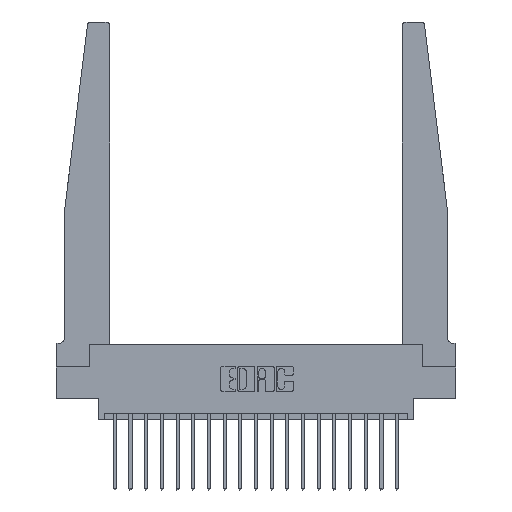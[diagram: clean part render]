
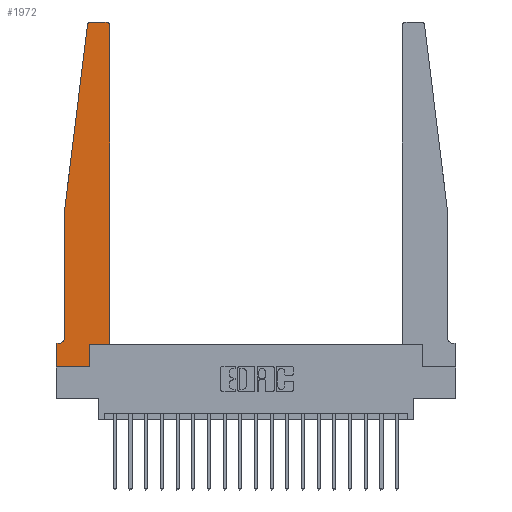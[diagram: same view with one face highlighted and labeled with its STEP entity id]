
A CAD part, top view. The second image highlights one B-rep face of the part: STEP entity #1972.
In plain terms, the highlighted planar face has unit normal (0, 0, 1).
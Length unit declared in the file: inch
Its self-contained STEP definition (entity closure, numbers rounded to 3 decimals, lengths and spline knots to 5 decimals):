
#54 = DIRECTION ( 'NONE',  ( 0., 0., -1. ) ) ;
#365 = VECTOR ( 'NONE', #19002, 39.37008 ) ;
#489 = EDGE_CURVE ( 'NONE', #7685, #6368, #19296, .T. ) ;
#491 = ORIENTED_EDGE ( 'NONE', *, *, #8057, .T. ) ;
#552 = VERTEX_POINT ( 'NONE', #6301 ) ;
#1669 = VECTOR ( 'NONE', #11376, 39.37008 ) ;
#1689 = CIRCLE ( 'NONE', #13489, 0.03 ) ;
#1708 = ORIENTED_EDGE ( 'NONE', *, *, #7081, .T. ) ;
#1972 = ADVANCED_FACE ( 'NONE', ( #8333 ), #5580, .T. ) ;
#2546 = VECTOR ( 'NONE', #20139, 39.37008 ) ;
#2625 = LINE ( 'NONE', #5913, #5986 ) ;
#2840 = VERTEX_POINT ( 'NONE', #19584 ) ;
#2884 = DIRECTION ( 'NONE',  ( -1., 0., 0. ) ) ;
#3231 = CARTESIAN_POINT ( 'NONE',  ( 0.425, 0.18, 0.37 ) ) ;
#3597 = CARTESIAN_POINT ( 'NONE',  ( 0.2605, 0.18, 0.37 ) ) ;
#3996 = LINE ( 'NONE', #17081, #2546 ) ;
#4361 = LINE ( 'NONE', #10800, #10312 ) ;
#4417 = CARTESIAN_POINT ( 'NONE',  ( 0., 0., 0.37 ) ) ;
#4528 = ORIENTED_EDGE ( 'NONE', *, *, #9600, .T. ) ;
#4577 = CARTESIAN_POINT ( 'NONE',  ( 0., 0., 0.37 ) ) ;
#4673 = CARTESIAN_POINT ( 'NONE',  ( 0.065, 0.1875, 0.37 ) ) ;
#4775 = DIRECTION ( 'NONE',  ( 0., 0., 1. ) ) ;
#4909 = CARTESIAN_POINT ( 'NONE',  ( 0.425, 0.18, 0.37 ) ) ;
#5580 = PLANE ( 'NONE',  #10446 ) ;
#5716 = VERTEX_POINT ( 'NONE', #14068 ) ;
#5913 = CARTESIAN_POINT ( 'NONE',  ( 0.065, 1.25, 0.37 ) ) ;
#5986 = VECTOR ( 'NONE', #12377, 39.37008 ) ;
#6007 = VERTEX_POINT ( 'NONE', #3597 ) ;
#6041 = ORIENTED_EDGE ( 'NONE', *, *, #489, .T. ) ;
#6210 = CARTESIAN_POINT ( 'NONE',  ( 0.2605, 0.18, 0.37 ) ) ;
#6301 = CARTESIAN_POINT ( 'NONE',  ( 0.2605, 0., 0.37 ) ) ;
#6368 = VERTEX_POINT ( 'NONE', #11832 ) ;
#7060 = ORIENTED_EDGE ( 'NONE', *, *, #12324, .T. ) ;
#7081 = EDGE_CURVE ( 'NONE', #10481, #552, #4361, .T. ) ;
#7345 = CARTESIAN_POINT ( 'NONE',  ( 0.24675, 2.72367, 0.37 ) ) ;
#7509 = EDGE_CURVE ( 'NONE', #13075, #10885, #2625, .T. ) ;
#7621 = DIRECTION ( 'NONE',  ( 1., 0., 0. ) ) ;
#7685 = VERTEX_POINT ( 'NONE', #16365 ) ;
#7714 = ORIENTED_EDGE ( 'NONE', *, *, #10382, .T. ) ;
#8057 = EDGE_CURVE ( 'NONE', #552, #6007, #17932, .T. ) ;
#8333 = FACE_OUTER_BOUND ( 'NONE', #13986, .T. ) ;
#8757 = ORIENTED_EDGE ( 'NONE', *, *, #17276, .T. ) ;
#8902 = ORIENTED_EDGE ( 'NONE', *, *, #13789, .T. ) ;
#8991 = VECTOR ( 'NONE', #9563, 39.37008 ) ;
#9555 = EDGE_CURVE ( 'NONE', #16680, #5716, #19242, .T. ) ;
#9563 = DIRECTION ( 'NONE',  ( 1., 0., 0. ) ) ;
#9600 = EDGE_CURVE ( 'NONE', #2840, #13075, #13892, .T. ) ;
#10312 = VECTOR ( 'NONE', #7621, 39.37008 ) ;
#10382 = EDGE_CURVE ( 'NONE', #10885, #17374, #3996, .T. ) ;
#10446 = AXIS2_PLACEMENT_3D ( 'NONE', #12041, #18467, #14779 ) ;
#10481 = VERTEX_POINT ( 'NONE', #4417 ) ;
#10800 = CARTESIAN_POINT ( 'NONE',  ( 0., 0., 0.37 ) ) ;
#10885 = VERTEX_POINT ( 'NONE', #14078 ) ;
#10942 = CARTESIAN_POINT ( 'NONE',  ( 0.395, 2.75, 0.37 ) ) ;
#11063 = DIRECTION ( 'NONE',  ( 0., 1., 0. ) ) ;
#11113 = DIRECTION ( 'NONE',  ( 1., 0., 0. ) ) ;
#11376 = DIRECTION ( 'NONE',  ( 0., 1., 0. ) ) ;
#11387 = AXIS2_PLACEMENT_3D ( 'NONE', #14527, #54, #2884 ) ;
#11805 = ORIENTED_EDGE ( 'NONE', *, *, #9555, .T. ) ;
#11832 = CARTESIAN_POINT ( 'NONE',  ( 0.425, 2.72, 0.37 ) ) ;
#12041 = CARTESIAN_POINT ( 'NONE',  ( 0., 0.1875, 0.37 ) ) ;
#12130 = CARTESIAN_POINT ( 'NONE',  ( 0.065, 0.2375, 0.37 ) ) ;
#12324 = EDGE_CURVE ( 'NONE', #17374, #16680, #18412, .T. ) ;
#12377 = DIRECTION ( 'NONE',  ( -0.122, -0.992, 0. ) ) ;
#12537 = ORIENTED_EDGE ( 'NONE', *, *, #7509, .T. ) ;
#12603 = CARTESIAN_POINT ( 'NONE',  ( 0.27653, 2.72, 0.37 ) ) ;
#12747 = LINE ( 'NONE', #4909, #8991 ) ;
#12805 = DIRECTION ( 'NONE',  ( 1., 0., 0. ) ) ;
#12891 = CARTESIAN_POINT ( 'NONE',  ( 0.25, 2.75, 0.37 ) ) ;
#13075 = VERTEX_POINT ( 'NONE', #7345 ) ;
#13082 = ORIENTED_EDGE ( 'NONE', *, *, #19927, .T. ) ;
#13284 = EDGE_CURVE ( 'NONE', #6007, #7685, #12747, .T. ) ;
#13489 = AXIS2_PLACEMENT_3D ( 'NONE', #17433, #16458, #12805 ) ;
#13598 = ORIENTED_EDGE ( 'NONE', *, *, #13284, .T. ) ;
#13789 = EDGE_CURVE ( 'NONE', #5716, #10481, #14403, .T. ) ;
#13892 = CIRCLE ( 'NONE', #16650, 0.03 ) ;
#13986 = EDGE_LOOP ( 'NONE', ( #13082, #4528, #12537, #7714, #7060, #11805, #8902, #1708, #491, #13598, #6041, #8757 ) ) ;
#14068 = CARTESIAN_POINT ( 'NONE',  ( 0., 0.1875, 0.37 ) ) ;
#14078 = CARTESIAN_POINT ( 'NONE',  ( 0.065, 1.25, 0.37 ) ) ;
#14403 = LINE ( 'NONE', #4577, #15766 ) ;
#14527 = CARTESIAN_POINT ( 'NONE',  ( 0.015, 0.2375, 0.37 ) ) ;
#14536 = VECTOR ( 'NONE', #11063, 39.37008 ) ;
#14634 = VERTEX_POINT ( 'NONE', #10942 ) ;
#14779 = DIRECTION ( 'NONE',  ( 1., 0., 0. ) ) ;
#15766 = VECTOR ( 'NONE', #15779, 39.37008 ) ;
#15779 = DIRECTION ( 'NONE',  ( 0., -1., 0. ) ) ;
#15825 = VECTOR ( 'NONE', #17658, 39.37008 ) ;
#16365 = CARTESIAN_POINT ( 'NONE',  ( 0.425, 0.18, 0.37 ) ) ;
#16458 = DIRECTION ( 'NONE',  ( 0., 0., 1. ) ) ;
#16650 = AXIS2_PLACEMENT_3D ( 'NONE', #12603, #4775, #11113 ) ;
#16680 = VERTEX_POINT ( 'NONE', #16935 ) ;
#16935 = CARTESIAN_POINT ( 'NONE',  ( 0.015, 0.1875, 0.37 ) ) ;
#17081 = CARTESIAN_POINT ( 'NONE',  ( 0.065, 1.25, 0.37 ) ) ;
#17276 = EDGE_CURVE ( 'NONE', #6368, #14634, #1689, .T. ) ;
#17374 = VERTEX_POINT ( 'NONE', #12130 ) ;
#17433 = CARTESIAN_POINT ( 'NONE',  ( 0.395, 2.72, 0.37 ) ) ;
#17658 = DIRECTION ( 'NONE',  ( -1., 0., 0. ) ) ;
#17845 = LINE ( 'NONE', #12891, #365 ) ;
#17932 = LINE ( 'NONE', #6210, #14536 ) ;
#18412 = CIRCLE ( 'NONE', #11387, 0.05 ) ;
#18467 = DIRECTION ( 'NONE',  ( 0., 0., 1. ) ) ;
#19002 = DIRECTION ( 'NONE',  ( -1., 0., 0. ) ) ;
#19242 = LINE ( 'NONE', #4673, #15825 ) ;
#19296 = LINE ( 'NONE', #3231, #1669 ) ;
#19584 = CARTESIAN_POINT ( 'NONE',  ( 0.27653, 2.75, 0.37 ) ) ;
#19927 = EDGE_CURVE ( 'NONE', #14634, #2840, #17845, .T. ) ;
#20139 = DIRECTION ( 'NONE',  ( 0., -1., 0. ) ) ;
